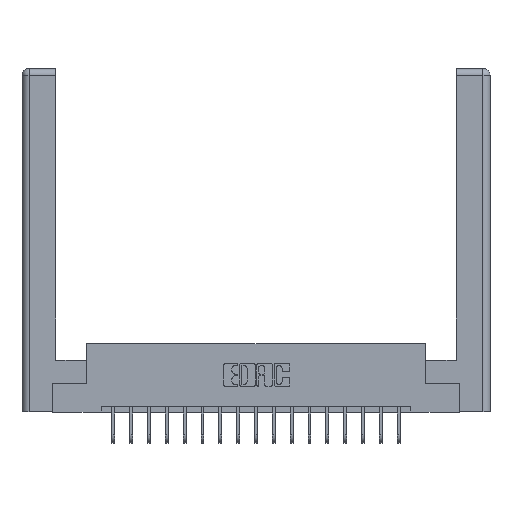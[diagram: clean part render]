
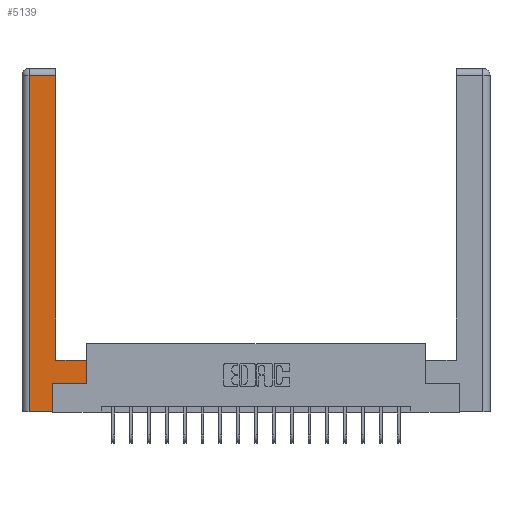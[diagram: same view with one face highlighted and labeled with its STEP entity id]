
A CAD part, top view. The second image highlights one B-rep face of the part: STEP entity #5139.
In plain terms, the highlighted planar face has unit normal (0, 0, 1).
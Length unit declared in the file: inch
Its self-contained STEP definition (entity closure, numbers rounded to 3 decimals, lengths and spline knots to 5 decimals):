
#43 = ORIENTED_EDGE ( 'NONE', *, *, #9672, .T. ) ;
#811 = DIRECTION ( 'NONE',  ( -1., 0., 0. ) ) ;
#1345 = CARTESIAN_POINT ( 'NONE',  ( 0.0615, 0., 0. ) ) ;
#1847 = CARTESIAN_POINT ( 'NONE',  ( 0.295, 2.94, 0. ) ) ;
#1944 = CARTESIAN_POINT ( 'NONE',  ( 0.0615, 2.94, 0. ) ) ;
#2110 = CARTESIAN_POINT ( 'NONE',  ( 0.265, 0., 0. ) ) ;
#2709 = CARTESIAN_POINT ( 'NONE',  ( 0.565, 0.245, 0. ) ) ;
#3282 = LINE ( 'NONE', #18891, #12602 ) ;
#3931 = VECTOR ( 'NONE', #5356, 39.37008 ) ;
#4494 = DIRECTION ( 'NONE',  ( 0., 1., 0. ) ) ;
#5056 = EDGE_CURVE ( 'NONE', #7761, #13637, #7892, .T. ) ;
#5087 = DIRECTION ( 'NONE',  ( -1., 0., 0. ) ) ;
#5139 = ADVANCED_FACE ( 'NONE', ( #14606 ), #9861, .F. ) ;
#5356 = DIRECTION ( 'NONE',  ( 1., 0., 0. ) ) ;
#5481 = LINE ( 'NONE', #18145, #3931 ) ;
#5639 = EDGE_CURVE ( 'NONE', #10743, #12587, #3282, .T. ) ;
#5666 = LINE ( 'NONE', #16857, #15695 ) ;
#6294 = VERTEX_POINT ( 'NONE', #2709 ) ;
#7609 = DIRECTION ( 'NONE',  ( -1., 0., 0. ) ) ;
#7761 = VERTEX_POINT ( 'NONE', #2110 ) ;
#7892 = LINE ( 'NONE', #16242, #17204 ) ;
#8130 = DIRECTION ( 'NONE',  ( 0., 0., -1. ) ) ;
#8189 = DIRECTION ( 'NONE',  ( 0., 1., 0. ) ) ;
#8550 = CARTESIAN_POINT ( 'NONE',  ( 0.565, 0.245, 0. ) ) ;
#8971 = LINE ( 'NONE', #10364, #15259 ) ;
#9264 = CARTESIAN_POINT ( 'NONE',  ( 0.295, 3., 0. ) ) ;
#9672 = EDGE_CURVE ( 'NONE', #20316, #7761, #5481, .T. ) ;
#9768 = ORIENTED_EDGE ( 'NONE', *, *, #5056, .T. ) ;
#9861 = PLANE ( 'NONE',  #14102 ) ;
#10229 = DIRECTION ( 'NONE',  ( 0., -1., 0. ) ) ;
#10323 = ORIENTED_EDGE ( 'NONE', *, *, #11272, .T. ) ;
#10364 = CARTESIAN_POINT ( 'NONE',  ( 0.0615, 2.94, 0. ) ) ;
#10743 = VERTEX_POINT ( 'NONE', #11957 ) ;
#11191 = ORIENTED_EDGE ( 'NONE', *, *, #14132, .T. ) ;
#11230 = CARTESIAN_POINT ( 'NONE',  ( 0.565, 0.45, 0. ) ) ;
#11272 = EDGE_CURVE ( 'NONE', #13637, #6294, #18217, .T. ) ;
#11488 = EDGE_LOOP ( 'NONE', ( #20398, #12866, #16985, #43, #9768, #10323, #11191, #12241 ) ) ;
#11566 = VECTOR ( 'NONE', #15994, 39.37008 ) ;
#11826 = DIRECTION ( 'NONE',  ( 1., 0., 0. ) ) ;
#11897 = VECTOR ( 'NONE', #11826, 39.37008 ) ;
#11957 = CARTESIAN_POINT ( 'NONE',  ( 0.565, 0.45, 0. ) ) ;
#12038 = EDGE_CURVE ( 'NONE', #12587, #16139, #16941, .T. ) ;
#12241 = ORIENTED_EDGE ( 'NONE', *, *, #5639, .T. ) ;
#12587 = VERTEX_POINT ( 'NONE', #20537 ) ;
#12602 = VECTOR ( 'NONE', #7609, 39.37008 ) ;
#12866 = ORIENTED_EDGE ( 'NONE', *, *, #16323, .T. ) ;
#13637 = VERTEX_POINT ( 'NONE', #18605 ) ;
#14102 = AXIS2_PLACEMENT_3D ( 'NONE', #14685, #8130, #5087 ) ;
#14132 = EDGE_CURVE ( 'NONE', #6294, #10743, #14589, .T. ) ;
#14589 = LINE ( 'NONE', #11230, #11566 ) ;
#14606 = FACE_OUTER_BOUND ( 'NONE', #11488, .T. ) ;
#14685 = CARTESIAN_POINT ( 'NONE',  ( 0., 0., 0. ) ) ;
#15259 = VECTOR ( 'NONE', #811, 39.37008 ) ;
#15695 = VECTOR ( 'NONE', #10229, 39.37008 ) ;
#15900 = VECTOR ( 'NONE', #4494, 39.37008 ) ;
#15994 = DIRECTION ( 'NONE',  ( 0., 1., 0. ) ) ;
#16139 = VERTEX_POINT ( 'NONE', #1847 ) ;
#16242 = CARTESIAN_POINT ( 'NONE',  ( 0.265, 0.245, 0. ) ) ;
#16323 = EDGE_CURVE ( 'NONE', #16139, #18876, #8971, .T. ) ;
#16857 = CARTESIAN_POINT ( 'NONE',  ( 0.0615, 0., 0. ) ) ;
#16941 = LINE ( 'NONE', #9264, #15900 ) ;
#16985 = ORIENTED_EDGE ( 'NONE', *, *, #18367, .T. ) ;
#17204 = VECTOR ( 'NONE', #8189, 39.37008 ) ;
#18145 = CARTESIAN_POINT ( 'NONE',  ( 0.265, 0., 0. ) ) ;
#18217 = LINE ( 'NONE', #8550, #11897 ) ;
#18367 = EDGE_CURVE ( 'NONE', #18876, #20316, #5666, .T. ) ;
#18605 = CARTESIAN_POINT ( 'NONE',  ( 0.265, 0.245, 0. ) ) ;
#18876 = VERTEX_POINT ( 'NONE', #1944 ) ;
#18891 = CARTESIAN_POINT ( 'NONE',  ( 0.295, 0.45, 0. ) ) ;
#20316 = VERTEX_POINT ( 'NONE', #1345 ) ;
#20398 = ORIENTED_EDGE ( 'NONE', *, *, #12038, .T. ) ;
#20537 = CARTESIAN_POINT ( 'NONE',  ( 0.295, 0.45, 0. ) ) ;
